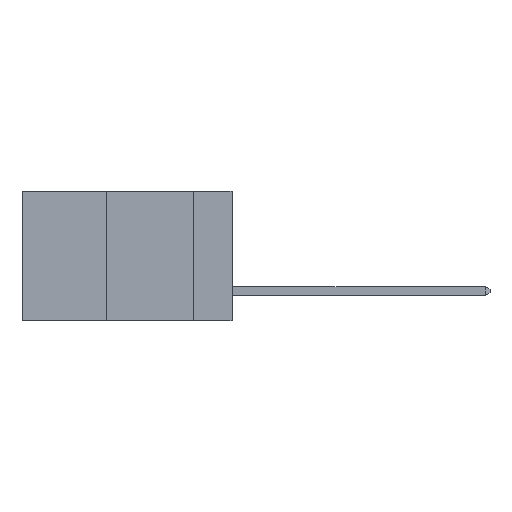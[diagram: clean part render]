
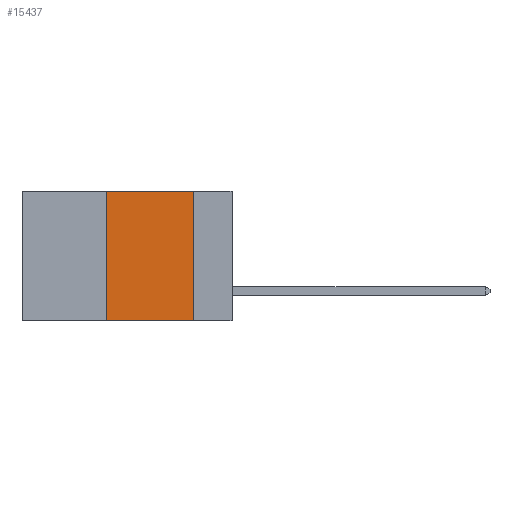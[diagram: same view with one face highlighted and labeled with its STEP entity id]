
A CAD part, left-side view. The second image highlights one B-rep face of the part: STEP entity #15437.
In plain terms, the highlighted planar face has unit normal (-1, 0, 0).
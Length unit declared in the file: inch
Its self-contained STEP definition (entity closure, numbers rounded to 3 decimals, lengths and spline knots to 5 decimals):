
#119 = AXIS2_PLACEMENT_3D ( 'NONE', #15766, #18490, #10243 ) ;
#435 = VERTEX_POINT ( 'NONE', #13983 ) ;
#1292 = VERTEX_POINT ( 'NONE', #12289 ) ;
#1743 = ORIENTED_EDGE ( 'NONE', *, *, #8121, .F. ) ;
#2546 = EDGE_LOOP ( 'NONE', ( #5194, #12783, #1743, #5627 ) ) ;
#5194 = ORIENTED_EDGE ( 'NONE', *, *, #12633, .F. ) ;
#5419 = DIRECTION ( 'NONE',  ( 0., -1., 0. ) ) ;
#5627 = ORIENTED_EDGE ( 'NONE', *, *, #15321, .T. ) ;
#5967 = VERTEX_POINT ( 'NONE', #11855 ) ;
#6518 = CARTESIAN_POINT ( 'NONE',  ( 0., 0.36, -0.37 ) ) ;
#7317 = LINE ( 'NONE', #13908, #14417 ) ;
#8121 = EDGE_CURVE ( 'NONE', #16320, #5967, #16392, .T. ) ;
#8971 = CARTESIAN_POINT ( 'NONE',  ( 0., 0.6, 0. ) ) ;
#10243 = DIRECTION ( 'NONE',  ( 0., 0., -1. ) ) ;
#10289 = VECTOR ( 'NONE', #17348, 39.37008 ) ;
#11250 = VECTOR ( 'NONE', #18456, 39.37008 ) ;
#11855 = CARTESIAN_POINT ( 'NONE',  ( 0., 0.36, 0. ) ) ;
#12289 = CARTESIAN_POINT ( 'NONE',  ( 0., 0.11, 0. ) ) ;
#12469 = CARTESIAN_POINT ( 'NONE',  ( 0., 0.36, 0. ) ) ;
#12633 = EDGE_CURVE ( 'NONE', #1292, #435, #18519, .T. ) ;
#12700 = FACE_OUTER_BOUND ( 'NONE', #2546, .T. ) ;
#12768 = VECTOR ( 'NONE', #15202, 39.37008 ) ;
#12783 = ORIENTED_EDGE ( 'NONE', *, *, #14569, .F. ) ;
#13908 = CARTESIAN_POINT ( 'NONE',  ( 0., 0.6, -0.37 ) ) ;
#13983 = CARTESIAN_POINT ( 'NONE',  ( 0., 0.11, -0.37 ) ) ;
#14004 = LINE ( 'NONE', #8971, #10289 ) ;
#14417 = VECTOR ( 'NONE', #5419, 39.37008 ) ;
#14569 = EDGE_CURVE ( 'NONE', #5967, #1292, #14004, .T. ) ;
#15202 = DIRECTION ( 'NONE',  ( 0., 0., 1. ) ) ;
#15321 = EDGE_CURVE ( 'NONE', #16320, #435, #7317, .T. ) ;
#15437 = ADVANCED_FACE ( 'NONE', ( #12700 ), #17158, .F. ) ;
#15766 = CARTESIAN_POINT ( 'NONE',  ( 0., 0.6, 0. ) ) ;
#16320 = VERTEX_POINT ( 'NONE', #6518 ) ;
#16392 = LINE ( 'NONE', #12469, #12768 ) ;
#17122 = CARTESIAN_POINT ( 'NONE',  ( 0., 0.11, 0. ) ) ;
#17158 = PLANE ( 'NONE',  #119 ) ;
#17348 = DIRECTION ( 'NONE',  ( 0., -1., 0. ) ) ;
#18456 = DIRECTION ( 'NONE',  ( 0., 0., -1. ) ) ;
#18490 = DIRECTION ( 'NONE',  ( 1., 0., 0. ) ) ;
#18519 = LINE ( 'NONE', #17122, #11250 ) ;
